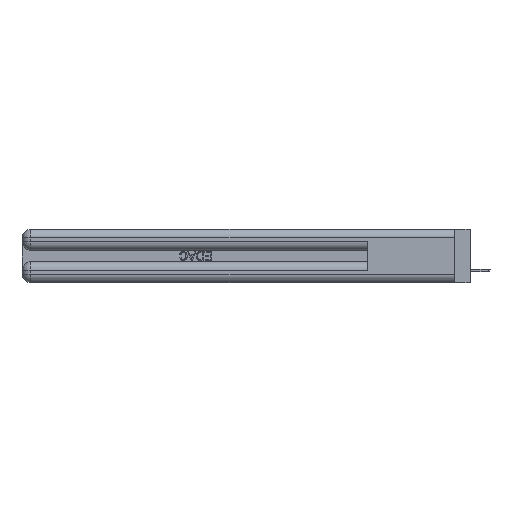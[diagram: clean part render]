
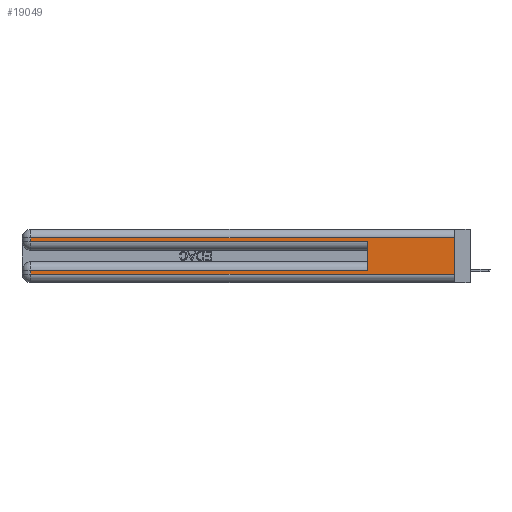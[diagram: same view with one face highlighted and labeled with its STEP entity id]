
A CAD part, left-side view. The second image highlights one B-rep face of the part: STEP entity #19049.
In plain terms, the highlighted planar face has unit normal (-1, 0, 0).
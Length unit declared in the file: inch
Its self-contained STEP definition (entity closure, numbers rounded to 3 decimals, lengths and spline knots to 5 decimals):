
#708 = CARTESIAN_POINT ( 'NONE',  ( 0., 0.6, 0.145 ) ) ;
#849 = DIRECTION ( 'NONE',  ( 0., 0., -1. ) ) ;
#914 = DIRECTION ( 'NONE',  ( 0., 0., 1. ) ) ;
#1383 = CARTESIAN_POINT ( 'NONE',  ( 0., 0., 0.085 ) ) ;
#3726 = VECTOR ( 'NONE', #914, 39.37008 ) ;
#4079 = LINE ( 'NONE', #38111, #18563 ) ;
#4365 = VECTOR ( 'NONE', #14143, 39.37008 ) ;
#4738 = EDGE_CURVE ( 'NONE', #37008, #22610, #30036, .T. ) ;
#5209 = EDGE_CURVE ( 'NONE', #7746, #26116, #33840, .T. ) ;
#5334 = ORIENTED_EDGE ( 'NONE', *, *, #23782, .T. ) ;
#5941 = DIRECTION ( 'NONE',  ( 0., 1., 0. ) ) ;
#6553 = EDGE_CURVE ( 'NONE', #7683, #13039, #24581, .T. ) ;
#7683 = VERTEX_POINT ( 'NONE', #20065 ) ;
#7746 = VERTEX_POINT ( 'NONE', #29552 ) ;
#8808 = EDGE_CURVE ( 'NONE', #7683, #7746, #30263, .T. ) ;
#8898 = LINE ( 'NONE', #11787, #32967 ) ;
#10813 = EDGE_CURVE ( 'NONE', #30404, #13039, #27311, .T. ) ;
#11198 = EDGE_CURVE ( 'NONE', #37008, #23544, #19857, .T. ) ;
#11585 = DIRECTION ( 'NONE',  ( 0., 0., -1. ) ) ;
#11611 = CARTESIAN_POINT ( 'NONE',  ( 0., 0., 0.37 ) ) ;
#11787 = CARTESIAN_POINT ( 'NONE',  ( 0., 2.94, 0.37 ) ) ;
#12338 = CARTESIAN_POINT ( 'NONE',  ( 0., 0.6, 0.085 ) ) ;
#12591 = DIRECTION ( 'NONE',  ( 0., 0., -1. ) ) ;
#13039 = VERTEX_POINT ( 'NONE', #32809 ) ;
#13474 = CARTESIAN_POINT ( 'NONE',  ( 0., 0.6, 0.285 ) ) ;
#13974 = DIRECTION ( 'NONE',  ( 0., 1., 0. ) ) ;
#14057 = ORIENTED_EDGE ( 'NONE', *, *, #4738, .T. ) ;
#14124 = VECTOR ( 'NONE', #5941, 39.37008 ) ;
#14143 = DIRECTION ( 'NONE',  ( 0., -1., 0. ) ) ;
#14347 = CARTESIAN_POINT ( 'NONE',  ( 0., 0., 0.06 ) ) ;
#15395 = CARTESIAN_POINT ( 'NONE',  ( 0., 2.94, 0.06 ) ) ;
#17219 = ORIENTED_EDGE ( 'NONE', *, *, #11198, .F. ) ;
#17709 = EDGE_CURVE ( 'NONE', #22610, #30404, #8898, .T. ) ;
#18563 = VECTOR ( 'NONE', #22838, 39.37008 ) ;
#18573 = CARTESIAN_POINT ( 'NONE',  ( 0., 2.94, 0.37 ) ) ;
#19049 = ADVANCED_FACE ( 'NONE', ( #22877 ), #19386, .F. ) ;
#19386 = PLANE ( 'NONE',  #33062 ) ;
#19390 = VECTOR ( 'NONE', #13974, 39.37008 ) ;
#19857 = LINE ( 'NONE', #708, #3726 ) ;
#20065 = CARTESIAN_POINT ( 'NONE',  ( 0., 0., 0.31 ) ) ;
#22610 = VERTEX_POINT ( 'NONE', #39726 ) ;
#22838 = DIRECTION ( 'NONE',  ( 0., -1., 0. ) ) ;
#22877 = FACE_OUTER_BOUND ( 'NONE', #28961, .T. ) ;
#23057 = VECTOR ( 'NONE', #12591, 39.37008 ) ;
#23544 = VERTEX_POINT ( 'NONE', #13474 ) ;
#23782 = EDGE_CURVE ( 'NONE', #26116, #23544, #4079, .T. ) ;
#24581 = LINE ( 'NONE', #11611, #32061 ) ;
#25164 = CARTESIAN_POINT ( 'NONE',  ( 0., 0., 0.37 ) ) ;
#26116 = VERTEX_POINT ( 'NONE', #36633 ) ;
#27311 = LINE ( 'NONE', #14347, #4365 ) ;
#27662 = DIRECTION ( 'NONE',  ( 0., 0., -1. ) ) ;
#28961 = EDGE_LOOP ( 'NONE', ( #31072, #29455, #29666, #5334, #17219, #14057, #37759, #30557 ) ) ;
#29455 = ORIENTED_EDGE ( 'NONE', *, *, #8808, .T. ) ;
#29552 = CARTESIAN_POINT ( 'NONE',  ( 0., 2.94, 0.31 ) ) ;
#29666 = ORIENTED_EDGE ( 'NONE', *, *, #5209, .T. ) ;
#30036 = LINE ( 'NONE', #1383, #19390 ) ;
#30263 = LINE ( 'NONE', #34173, #14124 ) ;
#30404 = VERTEX_POINT ( 'NONE', #15395 ) ;
#30557 = ORIENTED_EDGE ( 'NONE', *, *, #10813, .T. ) ;
#31072 = ORIENTED_EDGE ( 'NONE', *, *, #6553, .F. ) ;
#31980 = DIRECTION ( 'NONE',  ( 1., 0., 0. ) ) ;
#32061 = VECTOR ( 'NONE', #27662, 39.37008 ) ;
#32809 = CARTESIAN_POINT ( 'NONE',  ( 0., 0., 0.06 ) ) ;
#32967 = VECTOR ( 'NONE', #11585, 39.37008 ) ;
#33062 = AXIS2_PLACEMENT_3D ( 'NONE', #25164, #31980, #849 ) ;
#33840 = LINE ( 'NONE', #18573, #23057 ) ;
#34173 = CARTESIAN_POINT ( 'NONE',  ( 0., 0., 0.31 ) ) ;
#36633 = CARTESIAN_POINT ( 'NONE',  ( 0., 2.94, 0.285 ) ) ;
#37008 = VERTEX_POINT ( 'NONE', #12338 ) ;
#37759 = ORIENTED_EDGE ( 'NONE', *, *, #17709, .T. ) ;
#38111 = CARTESIAN_POINT ( 'NONE',  ( 0., 0., 0.285 ) ) ;
#39726 = CARTESIAN_POINT ( 'NONE',  ( 0., 2.94, 0.085 ) ) ;
